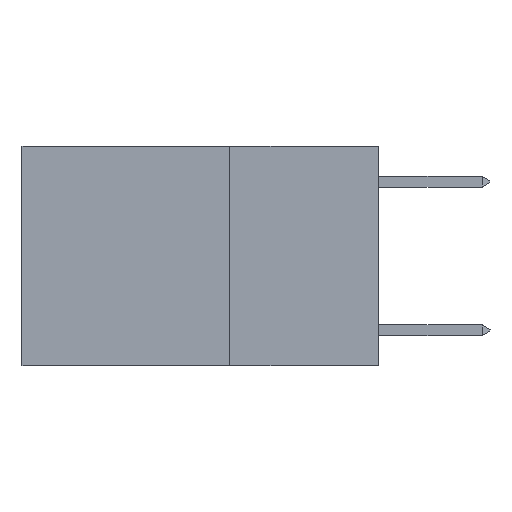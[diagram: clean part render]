
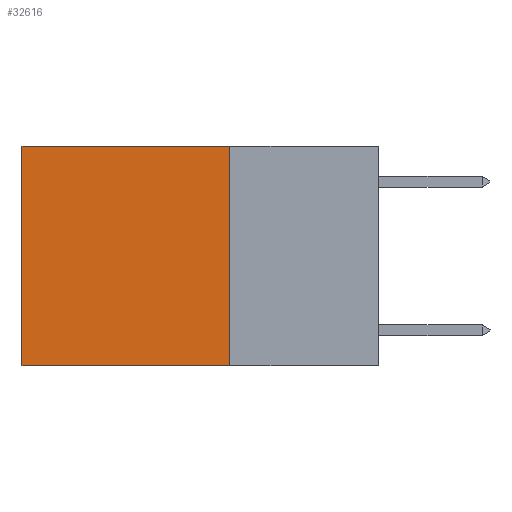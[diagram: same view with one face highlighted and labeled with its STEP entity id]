
A CAD part, left-side view. The second image highlights one B-rep face of the part: STEP entity #32616.
In plain terms, the highlighted planar face has unit normal (-1, 0, 0).
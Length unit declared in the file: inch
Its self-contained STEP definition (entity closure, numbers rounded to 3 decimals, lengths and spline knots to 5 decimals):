
#149 = CARTESIAN_POINT ( 'NONE',  ( 0.2625, 0.25, -0.37 ) ) ;
#623 = CARTESIAN_POINT ( 'NONE',  ( 0.2625, 0.25, 0. ) ) ;
#1006 = CARTESIAN_POINT ( 'NONE',  ( 0.2625, 0.6, 0. ) ) ;
#1351 = CARTESIAN_POINT ( 'NONE',  ( 0.2625, 0.25, 0. ) ) ;
#4513 = EDGE_CURVE ( 'NONE', #14741, #15644, #4711, .T. ) ;
#4711 = LINE ( 'NONE', #30514, #28256 ) ;
#5304 = LINE ( 'NONE', #5591, #13516 ) ;
#5591 = CARTESIAN_POINT ( 'NONE',  ( 0.2625, 0.25, 0. ) ) ;
#7581 = DIRECTION ( 'NONE',  ( 0., 1., 0. ) ) ;
#10852 = VECTOR ( 'NONE', #19173, 39.37008 ) ;
#12805 = DIRECTION ( 'NONE',  ( 0., 0., -1. ) ) ;
#12972 = VECTOR ( 'NONE', #7581, 39.37008 ) ;
#13516 = VECTOR ( 'NONE', #12805, 39.37008 ) ;
#13745 = ORIENTED_EDGE ( 'NONE', *, *, #17406, .T. ) ;
#14741 = VERTEX_POINT ( 'NONE', #149 ) ;
#14921 = LINE ( 'NONE', #27883, #12972 ) ;
#15644 = VERTEX_POINT ( 'NONE', #23227 ) ;
#16361 = EDGE_CURVE ( 'NONE', #26137, #14741, #5304, .T. ) ;
#17406 = EDGE_CURVE ( 'NONE', #26137, #30674, #14921, .T. ) ;
#19173 = DIRECTION ( 'NONE',  ( 0., 0., -1. ) ) ;
#22181 = EDGE_LOOP ( 'NONE', ( #24190, #28264, #27925, #13745 ) ) ;
#23227 = CARTESIAN_POINT ( 'NONE',  ( 0.2625, 0.6, -0.37 ) ) ;
#23330 = EDGE_CURVE ( 'NONE', #30674, #15644, #31872, .T. ) ;
#23841 = CARTESIAN_POINT ( 'NONE',  ( 0.2625, 0.6, 0. ) ) ;
#24190 = ORIENTED_EDGE ( 'NONE', *, *, #23330, .T. ) ;
#24313 = FACE_OUTER_BOUND ( 'NONE', #22181, .T. ) ;
#26137 = VERTEX_POINT ( 'NONE', #623 ) ;
#26500 = DIRECTION ( 'NONE',  ( 1., 0., 0. ) ) ;
#27652 = AXIS2_PLACEMENT_3D ( 'NONE', #1351, #26500, #29176 ) ;
#27883 = CARTESIAN_POINT ( 'NONE',  ( 0.2625, 0.25, 0. ) ) ;
#27925 = ORIENTED_EDGE ( 'NONE', *, *, #16361, .F. ) ;
#28256 = VECTOR ( 'NONE', #31008, 39.37008 ) ;
#28264 = ORIENTED_EDGE ( 'NONE', *, *, #4513, .F. ) ;
#29176 = DIRECTION ( 'NONE',  ( 0., 0., -1. ) ) ;
#30514 = CARTESIAN_POINT ( 'NONE',  ( 0.2625, 0.25, -0.37 ) ) ;
#30674 = VERTEX_POINT ( 'NONE', #1006 ) ;
#31008 = DIRECTION ( 'NONE',  ( 0., 1., 0. ) ) ;
#31872 = LINE ( 'NONE', #23841, #10852 ) ;
#31993 = PLANE ( 'NONE',  #27652 ) ;
#32616 = ADVANCED_FACE ( 'NONE', ( #24313 ), #31993, .F. ) ;
